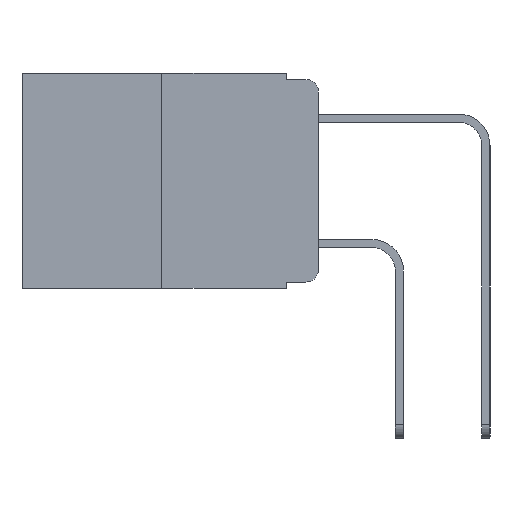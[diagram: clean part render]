
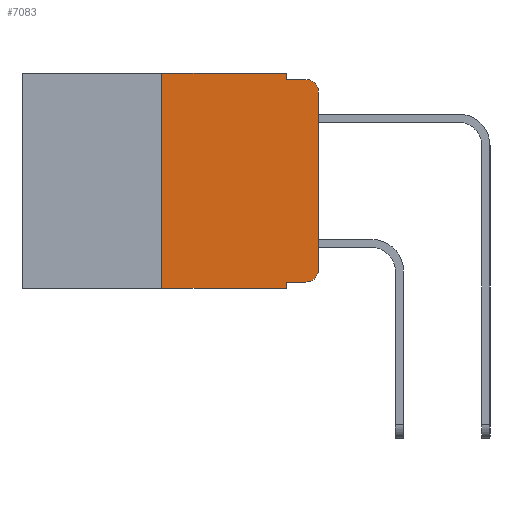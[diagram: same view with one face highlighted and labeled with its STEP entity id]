
A CAD part, left-side view. The second image highlights one B-rep face of the part: STEP entity #7083.
In plain terms, the highlighted planar face has unit normal (-1, 0, 0).
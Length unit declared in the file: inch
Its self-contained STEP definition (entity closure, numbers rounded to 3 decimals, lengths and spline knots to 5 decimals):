
#425 = VERTEX_POINT ( 'NONE', #3963 ) ;
#971 = LINE ( 'NONE', #12938, #11940 ) ;
#1046 = EDGE_CURVE ( 'NONE', #3934, #13790, #10018, .T. ) ;
#1407 = CARTESIAN_POINT ( 'NONE',  ( 0., 0.25, 0. ) ) ;
#1444 = EDGE_CURVE ( 'NONE', #7160, #425, #4178, .T. ) ;
#1703 = AXIS2_PLACEMENT_3D ( 'NONE', #5980, #5227, #5285 ) ;
#1959 = LINE ( 'NONE', #3674, #12462 ) ;
#1988 = VECTOR ( 'NONE', #7149, 39.37008 ) ;
#2154 = ORIENTED_EDGE ( 'NONE', *, *, #1444, .T. ) ;
#2196 = VECTOR ( 'NONE', #11641, 39.37008 ) ;
#2265 = DIRECTION ( 'NONE',  ( 0., -1., 0. ) ) ;
#2324 = CARTESIAN_POINT ( 'NONE',  ( 0., 0.473, 0. ) ) ;
#2402 = VECTOR ( 'NONE', #11449, 39.37008 ) ;
#2466 = EDGE_CURVE ( 'NONE', #13790, #5946, #16721, .T. ) ;
#2548 = VECTOR ( 'NONE', #5090, 39.37008 ) ;
#2668 = CARTESIAN_POINT ( 'NONE',  ( 0., 0.051, -0.333 ) ) ;
#3507 = CARTESIAN_POINT ( 'NONE',  ( 0., 0.02, -0.01 ) ) ;
#3653 = CARTESIAN_POINT ( 'NONE',  ( 0., 0.25, 0. ) ) ;
#3674 = CARTESIAN_POINT ( 'NONE',  ( 0., 0.473, 0. ) ) ;
#3732 = DIRECTION ( 'NONE',  ( 0., 0., -1. ) ) ;
#3823 = ORIENTED_EDGE ( 'NONE', *, *, #10682, .T. ) ;
#3839 = EDGE_CURVE ( 'NONE', #5946, #5338, #971, .T. ) ;
#3934 = VERTEX_POINT ( 'NONE', #2668 ) ;
#3963 = CARTESIAN_POINT ( 'NONE',  ( 0., 0.051, -0.343 ) ) ;
#4178 = LINE ( 'NONE', #14300, #7088 ) ;
#4921 = VERTEX_POINT ( 'NONE', #1407 ) ;
#5090 = DIRECTION ( 'NONE',  ( 0., 0., 1. ) ) ;
#5227 = DIRECTION ( 'NONE',  ( -1., 0., 0. ) ) ;
#5285 = DIRECTION ( 'NONE',  ( 0., 0., -1. ) ) ;
#5338 = VERTEX_POINT ( 'NONE', #18274 ) ;
#5391 = CIRCLE ( 'NONE', #9235, 0.02 ) ;
#5454 = DIRECTION ( 'NONE',  ( -1., 0., 0. ) ) ;
#5672 = EDGE_CURVE ( 'NONE', #14362, #18261, #13366, .T. ) ;
#5946 = VERTEX_POINT ( 'NONE', #8350 ) ;
#5980 = CARTESIAN_POINT ( 'NONE',  ( 0., 0.02, -0.313 ) ) ;
#6602 = ORIENTED_EDGE ( 'NONE', *, *, #2466, .T. ) ;
#7083 = ADVANCED_FACE ( 'NONE', ( #7670 ), #10870, .F. ) ;
#7088 = VECTOR ( 'NONE', #17368, 39.37008 ) ;
#7149 = DIRECTION ( 'NONE',  ( 0., -1., 0. ) ) ;
#7160 = VERTEX_POINT ( 'NONE', #18187 ) ;
#7477 = ORIENTED_EDGE ( 'NONE', *, *, #13156, .F. ) ;
#7670 = FACE_OUTER_BOUND ( 'NONE', #10626, .T. ) ;
#8350 = CARTESIAN_POINT ( 'NONE',  ( 0., 0., -0.313 ) ) ;
#9235 = AXIS2_PLACEMENT_3D ( 'NONE', #14035, #5454, #15467 ) ;
#10018 = LINE ( 'NONE', #13890, #1988 ) ;
#10140 = LINE ( 'NONE', #3653, #2548 ) ;
#10159 = EDGE_CURVE ( 'NONE', #18261, #11069, #16586, .T. ) ;
#10166 = CARTESIAN_POINT ( 'NONE',  ( 0., 0.02, -0.333 ) ) ;
#10192 = CARTESIAN_POINT ( 'NONE',  ( 0., 0.051, 0. ) ) ;
#10531 = ORIENTED_EDGE ( 'NONE', *, *, #5672, .F. ) ;
#10626 = EDGE_LOOP ( 'NONE', ( #11244, #3823, #13006, #10531, #12106, #17847, #2154, #7477, #18033, #6602 ) ) ;
#10682 = EDGE_CURVE ( 'NONE', #5338, #11069, #5391, .T. ) ;
#10870 = PLANE ( 'NONE',  #18331 ) ;
#11069 = VERTEX_POINT ( 'NONE', #3507 ) ;
#11186 = DIRECTION ( 'NONE',  ( 0., -1., 0. ) ) ;
#11244 = ORIENTED_EDGE ( 'NONE', *, *, #3839, .T. ) ;
#11449 = DIRECTION ( 'NONE',  ( 0., 0., -1. ) ) ;
#11641 = DIRECTION ( 'NONE',  ( 0., 0., -1. ) ) ;
#11940 = VECTOR ( 'NONE', #16906, 39.37008 ) ;
#12106 = ORIENTED_EDGE ( 'NONE', *, *, #13461, .F. ) ;
#12320 = DIRECTION ( 'NONE',  ( 1., 0., 0. ) ) ;
#12460 = CARTESIAN_POINT ( 'NONE',  ( 0., 0.051, 0. ) ) ;
#12462 = VECTOR ( 'NONE', #2265, 39.37008 ) ;
#12938 = CARTESIAN_POINT ( 'NONE',  ( 0., 0., 0. ) ) ;
#13006 = ORIENTED_EDGE ( 'NONE', *, *, #10159, .F. ) ;
#13092 = CARTESIAN_POINT ( 'NONE',  ( 0., 0.051, 0. ) ) ;
#13154 = CARTESIAN_POINT ( 'NONE',  ( 0., 0.051, -0.01 ) ) ;
#13156 = EDGE_CURVE ( 'NONE', #3934, #425, #13597, .T. ) ;
#13366 = LINE ( 'NONE', #12460, #2402 ) ;
#13461 = EDGE_CURVE ( 'NONE', #4921, #14362, #1959, .T. ) ;
#13597 = LINE ( 'NONE', #10192, #2196 ) ;
#13790 = VERTEX_POINT ( 'NONE', #10166 ) ;
#13890 = CARTESIAN_POINT ( 'NONE',  ( 0., 0.051, -0.333 ) ) ;
#14035 = CARTESIAN_POINT ( 'NONE',  ( 0., 0.02, -0.03 ) ) ;
#14300 = CARTESIAN_POINT ( 'NONE',  ( 0., 0.473, -0.343 ) ) ;
#14362 = VERTEX_POINT ( 'NONE', #13092 ) ;
#15467 = DIRECTION ( 'NONE',  ( 0., 0., -1. ) ) ;
#16083 = EDGE_CURVE ( 'NONE', #7160, #4921, #10140, .T. ) ;
#16129 = VECTOR ( 'NONE', #11186, 39.37008 ) ;
#16586 = LINE ( 'NONE', #16888, #16129 ) ;
#16721 = CIRCLE ( 'NONE', #1703, 0.02 ) ;
#16888 = CARTESIAN_POINT ( 'NONE',  ( 0., 0.051, -0.01 ) ) ;
#16906 = DIRECTION ( 'NONE',  ( 0., 0., 1. ) ) ;
#17368 = DIRECTION ( 'NONE',  ( 0., -1., 0. ) ) ;
#17847 = ORIENTED_EDGE ( 'NONE', *, *, #16083, .F. ) ;
#18033 = ORIENTED_EDGE ( 'NONE', *, *, #1046, .T. ) ;
#18187 = CARTESIAN_POINT ( 'NONE',  ( 0., 0.25, -0.343 ) ) ;
#18261 = VERTEX_POINT ( 'NONE', #13154 ) ;
#18274 = CARTESIAN_POINT ( 'NONE',  ( 0., 0., -0.03 ) ) ;
#18331 = AXIS2_PLACEMENT_3D ( 'NONE', #2324, #12320, #3732 ) ;
